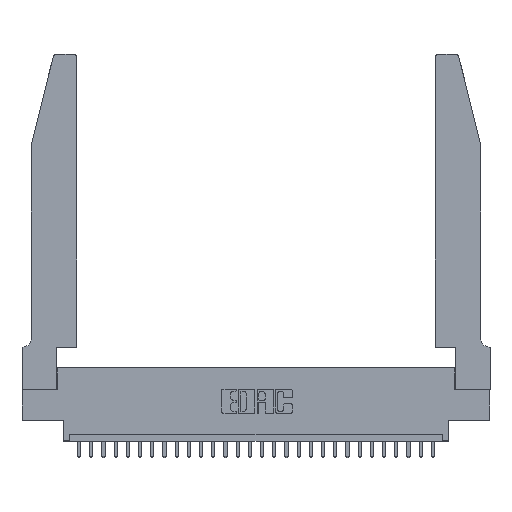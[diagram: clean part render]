
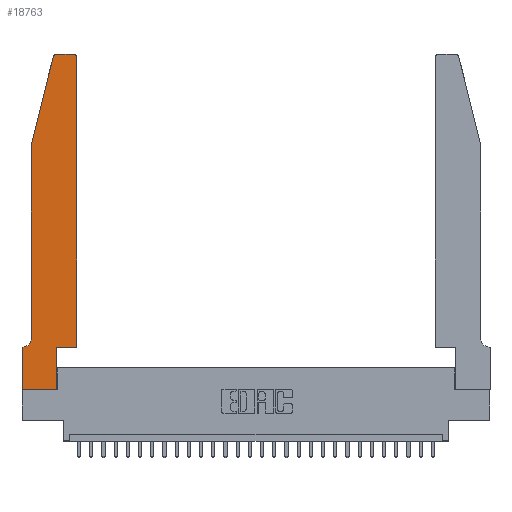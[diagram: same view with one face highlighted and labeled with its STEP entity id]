
A CAD part, top view. The second image highlights one B-rep face of the part: STEP entity #18763.
In plain terms, the highlighted planar face has unit normal (0, 0, 1).
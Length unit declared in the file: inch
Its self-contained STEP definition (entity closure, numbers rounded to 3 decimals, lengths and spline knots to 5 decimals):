
#341 = VERTEX_POINT ( 'NONE', #8781 ) ;
#348 = EDGE_CURVE ( 'NONE', #22445, #4115, #5233, .T. ) ;
#621 = ORIENTED_EDGE ( 'NONE', *, *, #15134, .T. ) ;
#1072 = EDGE_CURVE ( 'NONE', #22525, #7905, #2376, .T. ) ;
#1357 = AXIS2_PLACEMENT_3D ( 'NONE', #27786, #16537, #3158 ) ;
#2333 = LINE ( 'NONE', #17323, #29057 ) ;
#2376 = LINE ( 'NONE', #25682, #10778 ) ;
#2591 = CARTESIAN_POINT ( 'NONE',  ( 0.4505, 0.35, 0.37 ) ) ;
#2837 = CIRCLE ( 'NONE', #27404, 0.03 ) ;
#3158 = DIRECTION ( 'NONE',  ( 1., 0., 0. ) ) ;
#3791 = CARTESIAN_POINT ( 'NONE',  ( 0.0755, 0.42, 0.37 ) ) ;
#4103 = VERTEX_POINT ( 'NONE', #24718 ) ;
#4115 = VERTEX_POINT ( 'NONE', #13287 ) ;
#4385 = EDGE_LOOP ( 'NONE', ( #21551, #26337, #11911, #14038, #22011, #621, #9938, #17279, #5664, #28145, #24982, #12810 ) ) ;
#4475 = DIRECTION ( 'NONE',  ( 0., 0., 1. ) ) ;
#5155 = EDGE_CURVE ( 'NONE', #25784, #4103, #22051, .T. ) ;
#5182 = VERTEX_POINT ( 'NONE', #9066 ) ;
#5233 = LINE ( 'NONE', #2591, #12219 ) ;
#5564 = CARTESIAN_POINT ( 'NONE',  ( 0.0755, 2., 0.37 ) ) ;
#5664 = ORIENTED_EDGE ( 'NONE', *, *, #16957, .T. ) ;
#6004 = EDGE_CURVE ( 'NONE', #7905, #341, #11769, .T. ) ;
#6429 = CARTESIAN_POINT ( 'NONE',  ( 0.25487, 2.72718, 0.37 ) ) ;
#7638 = LINE ( 'NONE', #21073, #24872 ) ;
#7905 = VERTEX_POINT ( 'NONE', #3791 ) ;
#8781 = CARTESIAN_POINT ( 'NONE',  ( 0.0055, 0.35, 0.37 ) ) ;
#8927 = AXIS2_PLACEMENT_3D ( 'NONE', #17892, #18077, #15543 ) ;
#9066 = CARTESIAN_POINT ( 'NONE',  ( 0.4505, 2.72, 0.37 ) ) ;
#9938 = ORIENTED_EDGE ( 'NONE', *, *, #28881, .T. ) ;
#10327 = DIRECTION ( 'NONE',  ( 0., 1., 0. ) ) ;
#10413 = CARTESIAN_POINT ( 'NONE',  ( 0., 0.35, 0.37 ) ) ;
#10778 = VECTOR ( 'NONE', #12200, 39.37008 ) ;
#10785 = CARTESIAN_POINT ( 'NONE',  ( 0.0755, 2., 0.37 ) ) ;
#11038 = LINE ( 'NONE', #10785, #28273 ) ;
#11060 = EDGE_CURVE ( 'NONE', #15376, #22525, #11038, .T. ) ;
#11769 = CIRCLE ( 'NONE', #8927, 0.07 ) ;
#11911 = ORIENTED_EDGE ( 'NONE', *, *, #11060, .T. ) ;
#12041 = DIRECTION ( 'NONE',  ( 1., 0., 0. ) ) ;
#12048 = CARTESIAN_POINT ( 'NONE',  ( 0., 0., 0.37 ) ) ;
#12200 = DIRECTION ( 'NONE',  ( 0., -1., 0. ) ) ;
#12219 = VECTOR ( 'NONE', #18922, 39.37008 ) ;
#12621 = VERTEX_POINT ( 'NONE', #27562 ) ;
#12810 = ORIENTED_EDGE ( 'NONE', *, *, #26309, .T. ) ;
#13287 = CARTESIAN_POINT ( 'NONE',  ( 0.4505, 0.35, 0.37 ) ) ;
#13318 = DIRECTION ( 'NONE',  ( -0.239, -0.971, 0. ) ) ;
#13531 = LINE ( 'NONE', #12048, #22024 ) ;
#13561 = AXIS2_PLACEMENT_3D ( 'NONE', #28292, #4475, #17001 ) ;
#13805 = CARTESIAN_POINT ( 'NONE',  ( 0., 0., 0.37 ) ) ;
#13814 = VERTEX_POINT ( 'NONE', #10413 ) ;
#14038 = ORIENTED_EDGE ( 'NONE', *, *, #1072, .T. ) ;
#14273 = CIRCLE ( 'NONE', #13561, 0.03 ) ;
#14331 = VECTOR ( 'NONE', #27796, 39.37008 ) ;
#14611 = EDGE_CURVE ( 'NONE', #12621, #18531, #24928, .T. ) ;
#15134 = EDGE_CURVE ( 'NONE', #341, #13814, #7638, .T. ) ;
#15221 = EDGE_CURVE ( 'NONE', #18531, #15376, #14273, .T. ) ;
#15376 = VERTEX_POINT ( 'NONE', #6429 ) ;
#15492 = DIRECTION ( 'NONE',  ( 0., -1., 0. ) ) ;
#15543 = DIRECTION ( 'NONE',  ( -1., 0., 0. ) ) ;
#15629 = FACE_OUTER_BOUND ( 'NONE', #4385, .T. ) ;
#16302 = EDGE_CURVE ( 'NONE', #4115, #5182, #2333, .T. ) ;
#16537 = DIRECTION ( 'NONE',  ( 0., 0., 1. ) ) ;
#16735 = PLANE ( 'NONE',  #1357 ) ;
#16846 = CARTESIAN_POINT ( 'NONE',  ( 0., 0., 0.37 ) ) ;
#16957 = EDGE_CURVE ( 'NONE', #4103, #22445, #22659, .T. ) ;
#17001 = DIRECTION ( 'NONE',  ( 1., 0., 0. ) ) ;
#17279 = ORIENTED_EDGE ( 'NONE', *, *, #5155, .T. ) ;
#17323 = CARTESIAN_POINT ( 'NONE',  ( 0.4505, 0.35, 0.37 ) ) ;
#17892 = CARTESIAN_POINT ( 'NONE',  ( 0.0055, 0.42, 0.37 ) ) ;
#18077 = DIRECTION ( 'NONE',  ( 0., 0., -1. ) ) ;
#18531 = VERTEX_POINT ( 'NONE', #27119 ) ;
#18763 = ADVANCED_FACE ( 'NONE', ( #15629 ), #16735, .T. ) ;
#18922 = DIRECTION ( 'NONE',  ( 1., 0., 0. ) ) ;
#20203 = DIRECTION ( 'NONE',  ( 0., 1., 0. ) ) ;
#20818 = CARTESIAN_POINT ( 'NONE',  ( 0.2605, 2.75, 0.37 ) ) ;
#21073 = CARTESIAN_POINT ( 'NONE',  ( 0.0755, 0.35, 0.37 ) ) ;
#21551 = ORIENTED_EDGE ( 'NONE', *, *, #14611, .T. ) ;
#22011 = ORIENTED_EDGE ( 'NONE', *, *, #6004, .T. ) ;
#22024 = VECTOR ( 'NONE', #15492, 39.37008 ) ;
#22051 = LINE ( 'NONE', #13805, #23084 ) ;
#22445 = VERTEX_POINT ( 'NONE', #27490 ) ;
#22525 = VERTEX_POINT ( 'NONE', #5564 ) ;
#22659 = LINE ( 'NONE', #23729, #28285 ) ;
#23084 = VECTOR ( 'NONE', #27094, 39.37008 ) ;
#23729 = CARTESIAN_POINT ( 'NONE',  ( 0.2865, 0.35, 0.37 ) ) ;
#24718 = CARTESIAN_POINT ( 'NONE',  ( 0.2865, 0., 0.37 ) ) ;
#24872 = VECTOR ( 'NONE', #25706, 39.37008 ) ;
#24928 = LINE ( 'NONE', #20818, #14331 ) ;
#24982 = ORIENTED_EDGE ( 'NONE', *, *, #16302, .T. ) ;
#25425 = DIRECTION ( 'NONE',  ( 0., 0., 1. ) ) ;
#25682 = CARTESIAN_POINT ( 'NONE',  ( 0.0755, 2., 0.37 ) ) ;
#25706 = DIRECTION ( 'NONE',  ( -1., 0., 0. ) ) ;
#25784 = VERTEX_POINT ( 'NONE', #16846 ) ;
#26309 = EDGE_CURVE ( 'NONE', #5182, #12621, #2837, .T. ) ;
#26337 = ORIENTED_EDGE ( 'NONE', *, *, #15221, .T. ) ;
#27094 = DIRECTION ( 'NONE',  ( 1., 0., 0. ) ) ;
#27119 = CARTESIAN_POINT ( 'NONE',  ( 0.284, 2.75, 0.37 ) ) ;
#27404 = AXIS2_PLACEMENT_3D ( 'NONE', #27598, #25425, #12041 ) ;
#27490 = CARTESIAN_POINT ( 'NONE',  ( 0.2865, 0.35, 0.37 ) ) ;
#27562 = CARTESIAN_POINT ( 'NONE',  ( 0.4205, 2.75, 0.37 ) ) ;
#27598 = CARTESIAN_POINT ( 'NONE',  ( 0.4205, 2.72, 0.37 ) ) ;
#27786 = CARTESIAN_POINT ( 'NONE',  ( 0., 0.35, 0.37 ) ) ;
#27796 = DIRECTION ( 'NONE',  ( -1., 0., 0. ) ) ;
#28145 = ORIENTED_EDGE ( 'NONE', *, *, #348, .T. ) ;
#28273 = VECTOR ( 'NONE', #13318, 39.37008 ) ;
#28285 = VECTOR ( 'NONE', #10327, 39.37008 ) ;
#28292 = CARTESIAN_POINT ( 'NONE',  ( 0.284, 2.72, 0.37 ) ) ;
#28881 = EDGE_CURVE ( 'NONE', #13814, #25784, #13531, .T. ) ;
#29057 = VECTOR ( 'NONE', #20203, 39.37008 ) ;
